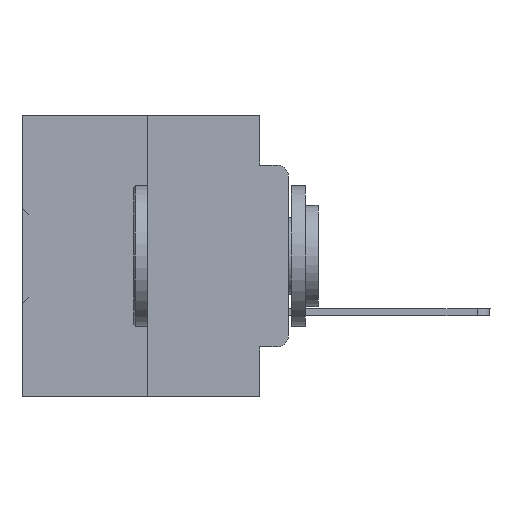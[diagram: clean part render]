
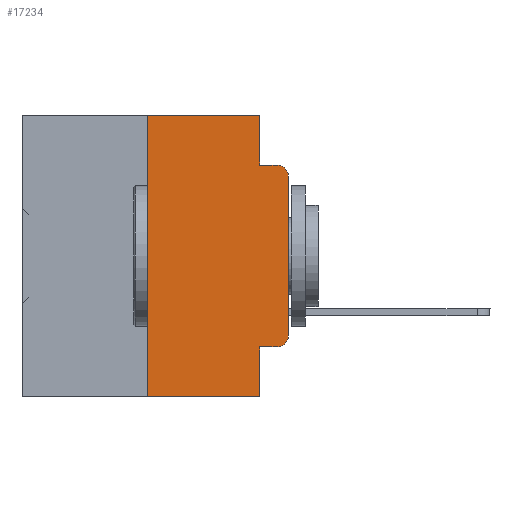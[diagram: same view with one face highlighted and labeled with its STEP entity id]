
A CAD part, left-side view. The second image highlights one B-rep face of the part: STEP entity #17234.
In plain terms, the highlighted planar face has unit normal (-1, 0, 0).
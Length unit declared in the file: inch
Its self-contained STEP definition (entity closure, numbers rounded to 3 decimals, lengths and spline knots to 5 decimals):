
#813 = ORIENTED_EDGE ( 'NONE', *, *, #25815, .F. ) ;
#849 = DIRECTION ( 'NONE',  ( 1., 0., 0. ) ) ;
#915 = CARTESIAN_POINT ( 'NONE',  ( 0., 0.25, 0. ) ) ;
#1966 = LINE ( 'NONE', #25925, #4261 ) ;
#2255 = ORIENTED_EDGE ( 'NONE', *, *, #5855, .T. ) ;
#2961 = CIRCLE ( 'NONE', #16005, 0.02 ) ;
#3636 = LINE ( 'NONE', #9300, #21546 ) ;
#3825 = ORIENTED_EDGE ( 'NONE', *, *, #19006, .T. ) ;
#3921 = CARTESIAN_POINT ( 'NONE',  ( 0., 0.02, -0.3915 ) ) ;
#4090 = VERTEX_POINT ( 'NONE', #37466 ) ;
#4261 = VECTOR ( 'NONE', #4865, 39.37008 ) ;
#4865 = DIRECTION ( 'NONE',  ( 0., -1., 0. ) ) ;
#5855 = EDGE_CURVE ( 'NONE', #26162, #18091, #35274, .T. ) ;
#8086 = CARTESIAN_POINT ( 'NONE',  ( 0., 0.02, -0.4115 ) ) ;
#8364 = LINE ( 'NONE', #29418, #32184 ) ;
#8490 = AXIS2_PLACEMENT_3D ( 'NONE', #3921, #18563, #31213 ) ;
#8504 = CARTESIAN_POINT ( 'NONE',  ( 0., 0., -0.1085 ) ) ;
#8713 = CARTESIAN_POINT ( 'NONE',  ( 0., 0.051, 0. ) ) ;
#8753 = ORIENTED_EDGE ( 'NONE', *, *, #31021, .T. ) ;
#8912 = VECTOR ( 'NONE', #34225, 39.37008 ) ;
#8916 = ORIENTED_EDGE ( 'NONE', *, *, #22448, .T. ) ;
#9144 = VERTEX_POINT ( 'NONE', #22003 ) ;
#9300 = CARTESIAN_POINT ( 'NONE',  ( 0., 0.051, 0. ) ) ;
#9388 = EDGE_CURVE ( 'NONE', #16732, #33502, #3636, .T. ) ;
#9389 = LINE ( 'NONE', #20920, #30308 ) ;
#9425 = VERTEX_POINT ( 'NONE', #915 ) ;
#9651 = CARTESIAN_POINT ( 'NONE',  ( 0., 0.051, -0.5 ) ) ;
#12600 = CARTESIAN_POINT ( 'NONE',  ( 0., 0.051, -0.4115 ) ) ;
#13602 = VECTOR ( 'NONE', #23231, 39.37008 ) ;
#13611 = ORIENTED_EDGE ( 'NONE', *, *, #9388, .F. ) ;
#13706 = LINE ( 'NONE', #32204, #13602 ) ;
#14109 = EDGE_CURVE ( 'NONE', #26162, #9425, #20616, .T. ) ;
#15477 = CARTESIAN_POINT ( 'NONE',  ( 0., 0.473, 0. ) ) ;
#16005 = AXIS2_PLACEMENT_3D ( 'NONE', #37031, #22601, #27869 ) ;
#16048 = FACE_OUTER_BOUND ( 'NONE', #20818, .T. ) ;
#16227 = CARTESIAN_POINT ( 'NONE',  ( 0., 0.473, -0.5 ) ) ;
#16732 = VERTEX_POINT ( 'NONE', #8713 ) ;
#17146 = DIRECTION ( 'NONE',  ( 0., 0., 1. ) ) ;
#17234 = ADVANCED_FACE ( 'NONE', ( #16048 ), #30475, .F. ) ;
#18075 = DIRECTION ( 'NONE',  ( 0., 0., 1. ) ) ;
#18091 = VERTEX_POINT ( 'NONE', #9651 ) ;
#18198 = DIRECTION ( 'NONE',  ( 0., -1., 0. ) ) ;
#18563 = DIRECTION ( 'NONE',  ( -1., 0., 0. ) ) ;
#19006 = EDGE_CURVE ( 'NONE', #4090, #29289, #21551, .T. ) ;
#19164 = DIRECTION ( 'NONE',  ( 0., -1., 0. ) ) ;
#20616 = LINE ( 'NONE', #24286, #26215 ) ;
#20818 = EDGE_LOOP ( 'NONE', ( #22979, #8753, #27861, #13611, #813, #28375, #2255, #36636, #3825, #8916 ) ) ;
#20920 = CARTESIAN_POINT ( 'NONE',  ( 0., 0.051, -0.0885 ) ) ;
#21546 = VECTOR ( 'NONE', #29980, 39.37008 ) ;
#21551 = LINE ( 'NONE', #12600, #8912 ) ;
#22003 = CARTESIAN_POINT ( 'NONE',  ( 0., 0.02, -0.0885 ) ) ;
#22448 = EDGE_CURVE ( 'NONE', #29289, #36903, #25304, .T. ) ;
#22601 = DIRECTION ( 'NONE',  ( -1., 0., 0. ) ) ;
#22636 = CARTESIAN_POINT ( 'NONE',  ( 0., 0.051, -0.0885 ) ) ;
#22979 = ORIENTED_EDGE ( 'NONE', *, *, #24120, .T. ) ;
#23231 = DIRECTION ( 'NONE',  ( 0., 0., -1. ) ) ;
#23945 = EDGE_CURVE ( 'NONE', #33502, #9144, #9389, .T. ) ;
#24120 = EDGE_CURVE ( 'NONE', #36903, #37576, #8364, .T. ) ;
#24286 = CARTESIAN_POINT ( 'NONE',  ( 0., 0.25, 0. ) ) ;
#24424 = DIRECTION ( 'NONE',  ( 0., 0., -1. ) ) ;
#25304 = CIRCLE ( 'NONE', #8490, 0.02 ) ;
#25352 = EDGE_CURVE ( 'NONE', #4090, #18091, #13706, .T. ) ;
#25815 = EDGE_CURVE ( 'NONE', #9425, #16732, #1966, .T. ) ;
#25925 = CARTESIAN_POINT ( 'NONE',  ( 0., 0.473, 0. ) ) ;
#26162 = VERTEX_POINT ( 'NONE', #31097 ) ;
#26215 = VECTOR ( 'NONE', #18075, 39.37008 ) ;
#27861 = ORIENTED_EDGE ( 'NONE', *, *, #23945, .F. ) ;
#27869 = DIRECTION ( 'NONE',  ( 0., 0., -1. ) ) ;
#28375 = ORIENTED_EDGE ( 'NONE', *, *, #14109, .F. ) ;
#29289 = VERTEX_POINT ( 'NONE', #8086 ) ;
#29418 = CARTESIAN_POINT ( 'NONE',  ( 0., 0., 0. ) ) ;
#29888 = CARTESIAN_POINT ( 'NONE',  ( 0., 0., -0.3915 ) ) ;
#29980 = DIRECTION ( 'NONE',  ( 0., 0., -1. ) ) ;
#29990 = AXIS2_PLACEMENT_3D ( 'NONE', #15477, #849, #24424 ) ;
#30308 = VECTOR ( 'NONE', #18198, 39.37008 ) ;
#30475 = PLANE ( 'NONE',  #29990 ) ;
#31021 = EDGE_CURVE ( 'NONE', #37576, #9144, #2961, .T. ) ;
#31097 = CARTESIAN_POINT ( 'NONE',  ( 0., 0.25, -0.5 ) ) ;
#31213 = DIRECTION ( 'NONE',  ( 0., 0., -1. ) ) ;
#32184 = VECTOR ( 'NONE', #17146, 39.37008 ) ;
#32204 = CARTESIAN_POINT ( 'NONE',  ( 0., 0.051, 0. ) ) ;
#33502 = VERTEX_POINT ( 'NONE', #22636 ) ;
#34225 = DIRECTION ( 'NONE',  ( 0., -1., 0. ) ) ;
#35274 = LINE ( 'NONE', #16227, #35728 ) ;
#35728 = VECTOR ( 'NONE', #19164, 39.37008 ) ;
#36636 = ORIENTED_EDGE ( 'NONE', *, *, #25352, .F. ) ;
#36903 = VERTEX_POINT ( 'NONE', #29888 ) ;
#37031 = CARTESIAN_POINT ( 'NONE',  ( 0., 0.02, -0.1085 ) ) ;
#37466 = CARTESIAN_POINT ( 'NONE',  ( 0., 0.051, -0.4115 ) ) ;
#37576 = VERTEX_POINT ( 'NONE', #8504 ) ;
